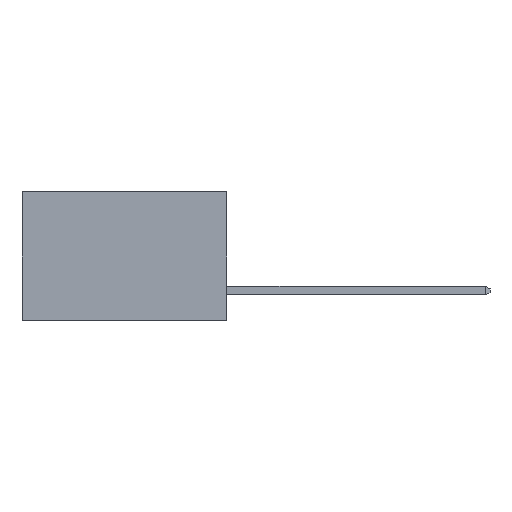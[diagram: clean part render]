
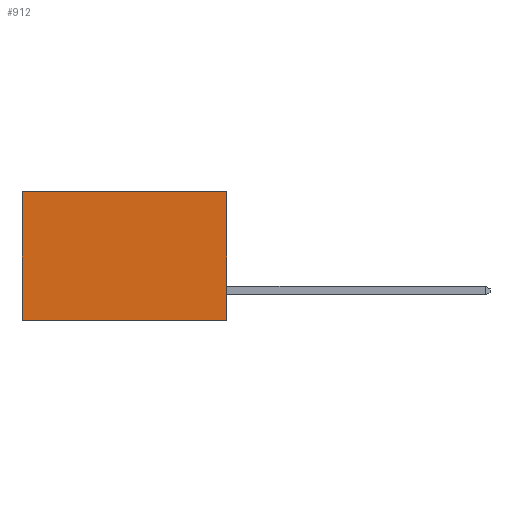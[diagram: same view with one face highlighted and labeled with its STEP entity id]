
A CAD part, left-side view. The second image highlights one B-rep face of the part: STEP entity #912.
In plain terms, the highlighted planar face has unit normal (-1, 0, 0).
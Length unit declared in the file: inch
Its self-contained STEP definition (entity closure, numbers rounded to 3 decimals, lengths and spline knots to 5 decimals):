
#572 = ORIENTED_EDGE ( 'NONE', *, *, #911, .F. ) ;
#704 = AXIS2_PLACEMENT_3D ( 'NONE', #5756, #6207, #7115 ) ;
#911 = EDGE_CURVE ( 'NONE', #1815, #2374, #4644, .T. ) ;
#912 = ADVANCED_FACE ( 'NONE', ( #12293 ), #9987, .F. ) ;
#1815 = VERTEX_POINT ( 'NONE', #3815 ) ;
#2195 = CARTESIAN_POINT ( 'NONE',  ( 0.277, 0.59, 0. ) ) ;
#2305 = VECTOR ( 'NONE', #4265, 39.37008 ) ;
#2374 = VERTEX_POINT ( 'NONE', #3717 ) ;
#2589 = VERTEX_POINT ( 'NONE', #11725 ) ;
#2800 = LINE ( 'NONE', #10864, #4470 ) ;
#3153 = ORIENTED_EDGE ( 'NONE', *, *, #11441, .T. ) ;
#3289 = CARTESIAN_POINT ( 'NONE',  ( 0.277, 0., 0. ) ) ;
#3717 = CARTESIAN_POINT ( 'NONE',  ( 0.277, 0., -0.37 ) ) ;
#3815 = CARTESIAN_POINT ( 'NONE',  ( 0.277, 0., 0. ) ) ;
#4253 = CARTESIAN_POINT ( 'NONE',  ( 0.277, 0., -0.37 ) ) ;
#4265 = DIRECTION ( 'NONE',  ( 0., 1., 0. ) ) ;
#4470 = VECTOR ( 'NONE', #10968, 39.37008 ) ;
#4644 = LINE ( 'NONE', #4253, #10025 ) ;
#4860 = LINE ( 'NONE', #3289, #2305 ) ;
#5118 = VERTEX_POINT ( 'NONE', #2195 ) ;
#5180 = EDGE_CURVE ( 'NONE', #2374, #2589, #8284, .T. ) ;
#5403 = ORIENTED_EDGE ( 'NONE', *, *, #9195, .T. ) ;
#5702 = VECTOR ( 'NONE', #12376, 39.37008 ) ;
#5756 = CARTESIAN_POINT ( 'NONE',  ( 0.277, 0., -0.37 ) ) ;
#5982 = EDGE_LOOP ( 'NONE', ( #5403, #10518, #572, #3153 ) ) ;
#6207 = DIRECTION ( 'NONE',  ( 1., 0., 0. ) ) ;
#7115 = DIRECTION ( 'NONE',  ( 0., 0., -1. ) ) ;
#8284 = LINE ( 'NONE', #11533, #5702 ) ;
#9195 = EDGE_CURVE ( 'NONE', #5118, #2589, #2800, .T. ) ;
#9987 = PLANE ( 'NONE',  #704 ) ;
#10025 = VECTOR ( 'NONE', #10973, 39.37008 ) ;
#10518 = ORIENTED_EDGE ( 'NONE', *, *, #5180, .F. ) ;
#10864 = CARTESIAN_POINT ( 'NONE',  ( 0.277, 0.59, -0.37 ) ) ;
#10968 = DIRECTION ( 'NONE',  ( 0., 0., -1. ) ) ;
#10973 = DIRECTION ( 'NONE',  ( 0., 0., -1. ) ) ;
#11441 = EDGE_CURVE ( 'NONE', #1815, #5118, #4860, .T. ) ;
#11533 = CARTESIAN_POINT ( 'NONE',  ( 0.277, 0., -0.37 ) ) ;
#11725 = CARTESIAN_POINT ( 'NONE',  ( 0.277, 0.59, -0.37 ) ) ;
#12293 = FACE_OUTER_BOUND ( 'NONE', #5982, .T. ) ;
#12376 = DIRECTION ( 'NONE',  ( 0., 1., 0. ) ) ;
